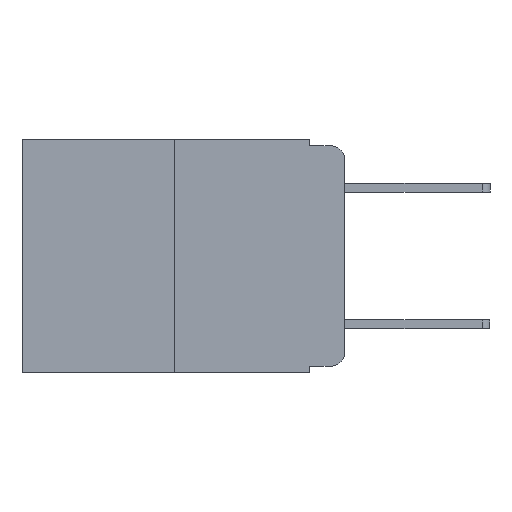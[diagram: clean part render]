
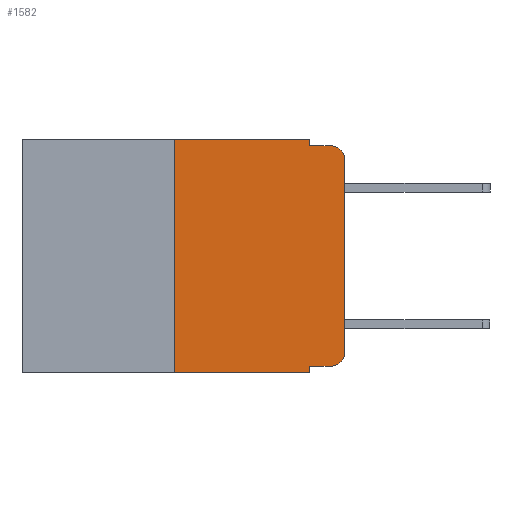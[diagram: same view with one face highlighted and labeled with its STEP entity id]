
A CAD part, left-side view. The second image highlights one B-rep face of the part: STEP entity #1582.
In plain terms, the highlighted planar face has unit normal (-1, 0, 0).
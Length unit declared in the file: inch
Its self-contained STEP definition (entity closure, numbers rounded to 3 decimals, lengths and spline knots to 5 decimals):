
#162 = VERTEX_POINT ( 'NONE', #2217 ) ;
#166 = VERTEX_POINT ( 'NONE', #2728 ) ;
#259 = EDGE_LOOP ( 'NONE', ( #5529, #16809, #9258, #14565, #3931, #17114, #1325, #1498, #2553, #8061 ) ) ;
#485 = EDGE_CURVE ( 'NONE', #12603, #11315, #8902, .T. ) ;
#513 = DIRECTION ( 'NONE',  ( -1., 0., 0. ) ) ;
#921 = CARTESIAN_POINT ( 'NONE',  ( 0., 0.051, -0.01 ) ) ;
#989 = PLANE ( 'NONE',  #14968 ) ;
#1140 = FACE_OUTER_BOUND ( 'NONE', #259, .T. ) ;
#1325 = ORIENTED_EDGE ( 'NONE', *, *, #3051, .T. ) ;
#1498 = ORIENTED_EDGE ( 'NONE', *, *, #7665, .F. ) ;
#1582 = ADVANCED_FACE ( 'NONE', ( #1140 ), #989, .F. ) ;
#1635 = CARTESIAN_POINT ( 'NONE',  ( 0., 0.051, 0. ) ) ;
#2217 = CARTESIAN_POINT ( 'NONE',  ( 0., 0.051, -0.343 ) ) ;
#2553 = ORIENTED_EDGE ( 'NONE', *, *, #14651, .T. ) ;
#2728 = CARTESIAN_POINT ( 'NONE',  ( 0., 0.25, -0.343 ) ) ;
#2885 = LINE ( 'NONE', #3027, #13473 ) ;
#3027 = CARTESIAN_POINT ( 'NONE',  ( 0., 0.25, 0. ) ) ;
#3051 = EDGE_CURVE ( 'NONE', #166, #162, #4903, .T. ) ;
#3131 = VECTOR ( 'NONE', #12959, 39.37008 ) ;
#3931 = ORIENTED_EDGE ( 'NONE', *, *, #9342, .F. ) ;
#4304 = CARTESIAN_POINT ( 'NONE',  ( 0., 0.051, -0.333 ) ) ;
#4903 = LINE ( 'NONE', #9571, #15052 ) ;
#5353 = VECTOR ( 'NONE', #11196, 39.37008 ) ;
#5529 = ORIENTED_EDGE ( 'NONE', *, *, #485, .T. ) ;
#6037 = LINE ( 'NONE', #11476, #9296 ) ;
#6094 = EDGE_CURVE ( 'NONE', #11329, #12603, #12328, .T. ) ;
#6510 = VECTOR ( 'NONE', #7117, 39.37008 ) ;
#6542 = CARTESIAN_POINT ( 'NONE',  ( 0., 0.02, -0.313 ) ) ;
#7104 = DIRECTION ( 'NONE',  ( 0., -1., 0. ) ) ;
#7117 = DIRECTION ( 'NONE',  ( 0., -1., 0. ) ) ;
#7166 = LINE ( 'NONE', #12252, #3131 ) ;
#7271 = DIRECTION ( 'NONE',  ( 0., 0., -1. ) ) ;
#7294 = CARTESIAN_POINT ( 'NONE',  ( 0., 0.051, 0. ) ) ;
#7334 = VERTEX_POINT ( 'NONE', #17527 ) ;
#7665 = EDGE_CURVE ( 'NONE', #13874, #162, #14825, .T. ) ;
#7899 = VECTOR ( 'NONE', #8178, 39.37008 ) ;
#8061 = ORIENTED_EDGE ( 'NONE', *, *, #6094, .T. ) ;
#8178 = DIRECTION ( 'NONE',  ( 0., 0., -1. ) ) ;
#8688 = CARTESIAN_POINT ( 'NONE',  ( 0., 0.02, -0.03 ) ) ;
#8898 = AXIS2_PLACEMENT_3D ( 'NONE', #8688, #513, #10095 ) ;
#8902 = LINE ( 'NONE', #12774, #15365 ) ;
#9172 = CARTESIAN_POINT ( 'NONE',  ( 0., 0., -0.313 ) ) ;
#9235 = CARTESIAN_POINT ( 'NONE',  ( 0., 0.25, 0. ) ) ;
#9258 = ORIENTED_EDGE ( 'NONE', *, *, #10959, .F. ) ;
#9296 = VECTOR ( 'NONE', #12890, 39.37008 ) ;
#9342 = EDGE_CURVE ( 'NONE', #13088, #10259, #7166, .T. ) ;
#9571 = CARTESIAN_POINT ( 'NONE',  ( 0., 0.473, -0.343 ) ) ;
#9741 = CIRCLE ( 'NONE', #8898, 0.02 ) ;
#10095 = DIRECTION ( 'NONE',  ( 0., 0., -1. ) ) ;
#10097 = DIRECTION ( 'NONE',  ( 0., 0., -1. ) ) ;
#10130 = DIRECTION ( 'NONE',  ( -1., 0., 0. ) ) ;
#10259 = VERTEX_POINT ( 'NONE', #1635 ) ;
#10737 = CARTESIAN_POINT ( 'NONE',  ( 0., 0.02, -0.333 ) ) ;
#10959 = EDGE_CURVE ( 'NONE', #12594, #7334, #17534, .T. ) ;
#10984 = EDGE_CURVE ( 'NONE', #166, #13088, #2885, .T. ) ;
#11196 = DIRECTION ( 'NONE',  ( 0., -1., 0. ) ) ;
#11315 = VERTEX_POINT ( 'NONE', #12115 ) ;
#11329 = VERTEX_POINT ( 'NONE', #10737 ) ;
#11345 = DIRECTION ( 'NONE',  ( 0., 0., 1. ) ) ;
#11476 = CARTESIAN_POINT ( 'NONE',  ( 0., 0.051, 0. ) ) ;
#12115 = CARTESIAN_POINT ( 'NONE',  ( 0., 0., -0.03 ) ) ;
#12174 = CARTESIAN_POINT ( 'NONE',  ( 0., 0.051, -0.333 ) ) ;
#12252 = CARTESIAN_POINT ( 'NONE',  ( 0., 0.473, 0. ) ) ;
#12328 = CIRCLE ( 'NONE', #17545, 0.02 ) ;
#12331 = EDGE_CURVE ( 'NONE', #11315, #7334, #9741, .T. ) ;
#12353 = EDGE_CURVE ( 'NONE', #10259, #12594, #6037, .T. ) ;
#12581 = DIRECTION ( 'NONE',  ( 0., 0., 1. ) ) ;
#12594 = VERTEX_POINT ( 'NONE', #921 ) ;
#12603 = VERTEX_POINT ( 'NONE', #9172 ) ;
#12774 = CARTESIAN_POINT ( 'NONE',  ( 0., 0., 0. ) ) ;
#12890 = DIRECTION ( 'NONE',  ( 0., 0., -1. ) ) ;
#12923 = LINE ( 'NONE', #4304, #5353 ) ;
#12959 = DIRECTION ( 'NONE',  ( 0., -1., 0. ) ) ;
#13088 = VERTEX_POINT ( 'NONE', #9235 ) ;
#13272 = CARTESIAN_POINT ( 'NONE',  ( 0., 0.473, 0. ) ) ;
#13469 = DIRECTION ( 'NONE',  ( 1., 0., 0. ) ) ;
#13473 = VECTOR ( 'NONE', #11345, 39.37008 ) ;
#13874 = VERTEX_POINT ( 'NONE', #12174 ) ;
#14565 = ORIENTED_EDGE ( 'NONE', *, *, #12353, .F. ) ;
#14651 = EDGE_CURVE ( 'NONE', #13874, #11329, #12923, .T. ) ;
#14825 = LINE ( 'NONE', #7294, #7899 ) ;
#14968 = AXIS2_PLACEMENT_3D ( 'NONE', #13272, #13469, #7271 ) ;
#15052 = VECTOR ( 'NONE', #7104, 39.37008 ) ;
#15365 = VECTOR ( 'NONE', #12581, 39.37008 ) ;
#16809 = ORIENTED_EDGE ( 'NONE', *, *, #12331, .T. ) ;
#16818 = CARTESIAN_POINT ( 'NONE',  ( 0., 0.051, -0.01 ) ) ;
#17114 = ORIENTED_EDGE ( 'NONE', *, *, #10984, .F. ) ;
#17527 = CARTESIAN_POINT ( 'NONE',  ( 0., 0.02, -0.01 ) ) ;
#17534 = LINE ( 'NONE', #16818, #6510 ) ;
#17545 = AXIS2_PLACEMENT_3D ( 'NONE', #6542, #10130, #10097 ) ;
